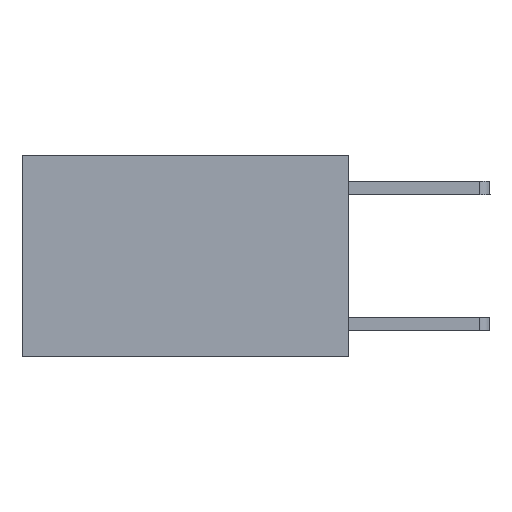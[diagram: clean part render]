
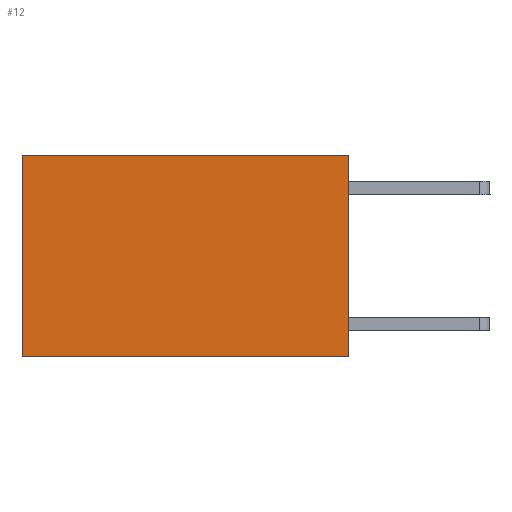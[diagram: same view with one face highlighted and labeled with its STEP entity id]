
A CAD part, left-side view. The second image highlights one B-rep face of the part: STEP entity #12.
In plain terms, the highlighted planar face has unit normal (-1, 0, 0).
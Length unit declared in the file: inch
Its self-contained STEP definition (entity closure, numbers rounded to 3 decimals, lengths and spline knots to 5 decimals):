
#12 = ADVANCED_FACE ( 'NONE', ( #267 ), #12453, .F. ) ;
#267 = FACE_OUTER_BOUND ( 'NONE', #8320, .T. ) ;
#375 = EDGE_CURVE ( 'NONE', #5069, #4309, #9855, .T. ) ;
#629 = CARTESIAN_POINT ( 'NONE',  ( 0.2625, 0., 0. ) ) ;
#964 = CARTESIAN_POINT ( 'NONE',  ( 0.2625, 0.6, -0.37 ) ) ;
#1071 = LINE ( 'NONE', #1518, #8828 ) ;
#1510 = LINE ( 'NONE', #5744, #4420 ) ;
#1518 = CARTESIAN_POINT ( 'NONE',  ( 0.2625, 0., 0. ) ) ;
#1616 = EDGE_CURVE ( 'NONE', #7494, #5069, #1071, .T. ) ;
#1753 = LINE ( 'NONE', #6074, #7112 ) ;
#1802 = CARTESIAN_POINT ( 'NONE',  ( 0.2625, 0., -0.37 ) ) ;
#2248 = CARTESIAN_POINT ( 'NONE',  ( 0.2625, 0.6, 0. ) ) ;
#3174 = CARTESIAN_POINT ( 'NONE',  ( 0.2625, 0., -0.37 ) ) ;
#4309 = VERTEX_POINT ( 'NONE', #964 ) ;
#4420 = VECTOR ( 'NONE', #12557, 39.37008 ) ;
#5069 = VERTEX_POINT ( 'NONE', #3174 ) ;
#5694 = CARTESIAN_POINT ( 'NONE',  ( 0.2625, 0., 0. ) ) ;
#5744 = CARTESIAN_POINT ( 'NONE',  ( 0.2625, 0.6, 0. ) ) ;
#6074 = CARTESIAN_POINT ( 'NONE',  ( 0.2625, 0., 0. ) ) ;
#7112 = VECTOR ( 'NONE', #9165, 39.37008 ) ;
#7163 = ORIENTED_EDGE ( 'NONE', *, *, #375, .F. ) ;
#7494 = VERTEX_POINT ( 'NONE', #629 ) ;
#7597 = ORIENTED_EDGE ( 'NONE', *, *, #9716, .T. ) ;
#8320 = EDGE_LOOP ( 'NONE', ( #11651, #7163, #8434, #7597 ) ) ;
#8434 = ORIENTED_EDGE ( 'NONE', *, *, #1616, .F. ) ;
#8514 = DIRECTION ( 'NONE',  ( 0., 1., 0. ) ) ;
#8828 = VECTOR ( 'NONE', #11959, 39.37008 ) ;
#9165 = DIRECTION ( 'NONE',  ( 0., 1., 0. ) ) ;
#9716 = EDGE_CURVE ( 'NONE', #7494, #12681, #1753, .T. ) ;
#9741 = VECTOR ( 'NONE', #8514, 39.37008 ) ;
#9855 = LINE ( 'NONE', #1802, #9741 ) ;
#9913 = DIRECTION ( 'NONE',  ( 1., 0., 0. ) ) ;
#11397 = EDGE_CURVE ( 'NONE', #12681, #4309, #1510, .T. ) ;
#11651 = ORIENTED_EDGE ( 'NONE', *, *, #11397, .T. ) ;
#11959 = DIRECTION ( 'NONE',  ( 0., 0., -1. ) ) ;
#12355 = AXIS2_PLACEMENT_3D ( 'NONE', #5694, #9913, #12665 ) ;
#12453 = PLANE ( 'NONE',  #12355 ) ;
#12557 = DIRECTION ( 'NONE',  ( 0., 0., -1. ) ) ;
#12665 = DIRECTION ( 'NONE',  ( 0., 0., -1. ) ) ;
#12681 = VERTEX_POINT ( 'NONE', #2248 ) ;
